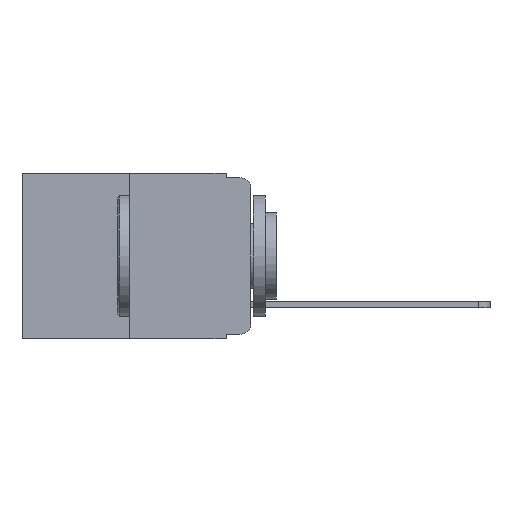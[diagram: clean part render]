
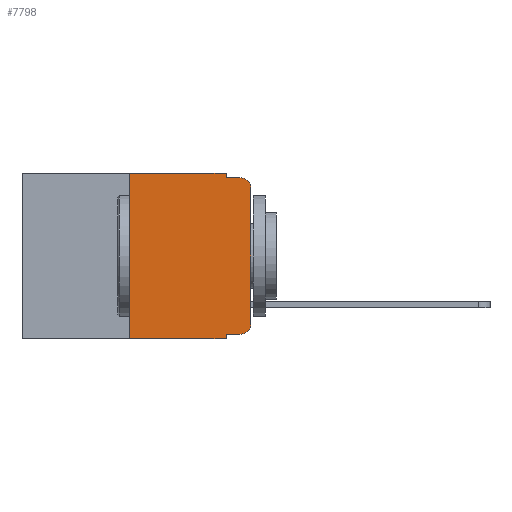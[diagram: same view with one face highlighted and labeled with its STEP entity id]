
A CAD part, left-side view. The second image highlights one B-rep face of the part: STEP entity #7798.
In plain terms, the highlighted planar face has unit normal (-1, 0, 0).
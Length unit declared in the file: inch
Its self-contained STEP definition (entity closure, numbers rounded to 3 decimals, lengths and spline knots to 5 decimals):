
#70 = DIRECTION ( 'NONE',  ( 0., 0., 1. ) ) ;
#279 = ORIENTED_EDGE ( 'NONE', *, *, #6738, .F. ) ;
#283 = CARTESIAN_POINT ( 'NONE',  ( 0., 0., 0. ) ) ;
#326 = EDGE_LOOP ( 'NONE', ( #13229, #1941, #5001, #279, #971, #1552, #1792, #2138, #4042, #7269 ) ) ;
#345 = VERTEX_POINT ( 'NONE', #1131 ) ;
#574 = CARTESIAN_POINT ( 'NONE',  ( 0., 0.051, -0.333 ) ) ;
#971 = ORIENTED_EDGE ( 'NONE', *, *, #5576, .F. ) ;
#1126 = EDGE_CURVE ( 'NONE', #345, #3323, #8335, .T. ) ;
#1131 = CARTESIAN_POINT ( 'NONE',  ( 0., 0.25, -0.343 ) ) ;
#1309 = VERTEX_POINT ( 'NONE', #3996 ) ;
#1339 = VERTEX_POINT ( 'NONE', #2635 ) ;
#1436 = CIRCLE ( 'NONE', #5843, 0.02 ) ;
#1552 = ORIENTED_EDGE ( 'NONE', *, *, #6776, .F. ) ;
#1668 = CIRCLE ( 'NONE', #12823, 0.02 ) ;
#1792 = ORIENTED_EDGE ( 'NONE', *, *, #1126, .T. ) ;
#1941 = ORIENTED_EDGE ( 'NONE', *, *, #6698, .T. ) ;
#2138 = ORIENTED_EDGE ( 'NONE', *, *, #6799, .F. ) ;
#2353 = DIRECTION ( 'NONE',  ( 0., -1., 0. ) ) ;
#2395 = DIRECTION ( 'NONE',  ( 1., 0., 0. ) ) ;
#2454 = VERTEX_POINT ( 'NONE', #9579 ) ;
#2459 = VERTEX_POINT ( 'NONE', #8147 ) ;
#2635 = CARTESIAN_POINT ( 'NONE',  ( 0., 0., -0.313 ) ) ;
#2829 = VERTEX_POINT ( 'NONE', #9335 ) ;
#3003 = VECTOR ( 'NONE', #8127, 39.37008 ) ;
#3323 = VERTEX_POINT ( 'NONE', #3618 ) ;
#3515 = DIRECTION ( 'NONE',  ( 0., 0., -1. ) ) ;
#3618 = CARTESIAN_POINT ( 'NONE',  ( 0., 0.051, -0.343 ) ) ;
#3692 = LINE ( 'NONE', #9010, #3003 ) ;
#3721 = DIRECTION ( 'NONE',  ( 0., -1., 0. ) ) ;
#3739 = CARTESIAN_POINT ( 'NONE',  ( 0., 0.051, 0. ) ) ;
#3996 = CARTESIAN_POINT ( 'NONE',  ( 0., 0.051, 0. ) ) ;
#4042 = ORIENTED_EDGE ( 'NONE', *, *, #6817, .T. ) ;
#4272 = VERTEX_POINT ( 'NONE', #6217 ) ;
#4340 = VERTEX_POINT ( 'NONE', #9428 ) ;
#4472 = CARTESIAN_POINT ( 'NONE',  ( 0., 0.473, 0. ) ) ;
#4518 = DIRECTION ( 'NONE',  ( 0., -1., 0. ) ) ;
#5001 = ORIENTED_EDGE ( 'NONE', *, *, #6722, .F. ) ;
#5290 = LINE ( 'NONE', #574, #12561 ) ;
#5558 = VECTOR ( 'NONE', #3721, 39.37008 ) ;
#5576 = EDGE_CURVE ( 'NONE', #2459, #1309, #8812, .T. ) ;
#5843 = AXIS2_PLACEMENT_3D ( 'NONE', #11190, #11175, #11147 ) ;
#6100 = VECTOR ( 'NONE', #4518, 39.37008 ) ;
#6217 = CARTESIAN_POINT ( 'NONE',  ( 0., 0.02, -0.01 ) ) ;
#6686 = EDGE_CURVE ( 'NONE', #1339, #2829, #10124, .T. ) ;
#6698 = EDGE_CURVE ( 'NONE', #2829, #4272, #1668, .T. ) ;
#6722 = EDGE_CURVE ( 'NONE', #4340, #4272, #11621, .T. ) ;
#6738 = EDGE_CURVE ( 'NONE', #1309, #4340, #8966, .T. ) ;
#6765 = CARTESIAN_POINT ( 'NONE',  ( 0., 0.473, 0. ) ) ;
#6776 = EDGE_CURVE ( 'NONE', #345, #2459, #3692, .T. ) ;
#6799 = EDGE_CURVE ( 'NONE', #6889, #3323, #13074, .T. ) ;
#6817 = EDGE_CURVE ( 'NONE', #6889, #2454, #5290, .T. ) ;
#6876 = EDGE_CURVE ( 'NONE', #2454, #1339, #1436, .T. ) ;
#6889 = VERTEX_POINT ( 'NONE', #11275 ) ;
#7269 = ORIENTED_EDGE ( 'NONE', *, *, #6876, .T. ) ;
#7657 = AXIS2_PLACEMENT_3D ( 'NONE', #6765, #2395, #9766 ) ;
#7798 = ADVANCED_FACE ( 'NONE', ( #8355 ), #8806, .F. ) ;
#8127 = DIRECTION ( 'NONE',  ( 0., 0., 1. ) ) ;
#8147 = CARTESIAN_POINT ( 'NONE',  ( 0., 0.25, 0. ) ) ;
#8335 = LINE ( 'NONE', #10536, #5558 ) ;
#8355 = FACE_OUTER_BOUND ( 'NONE', #326, .T. ) ;
#8806 = PLANE ( 'NONE',  #7657 ) ;
#8812 = LINE ( 'NONE', #4472, #6100 ) ;
#8966 = LINE ( 'NONE', #9173, #11332 ) ;
#9010 = CARTESIAN_POINT ( 'NONE',  ( 0., 0.25, 0. ) ) ;
#9173 = CARTESIAN_POINT ( 'NONE',  ( 0., 0.051, 0. ) ) ;
#9335 = CARTESIAN_POINT ( 'NONE',  ( 0., 0., -0.03 ) ) ;
#9377 = DIRECTION ( 'NONE',  ( 0., 0., -1. ) ) ;
#9428 = CARTESIAN_POINT ( 'NONE',  ( 0., 0.051, -0.01 ) ) ;
#9575 = VECTOR ( 'NONE', #10414, 39.37008 ) ;
#9579 = CARTESIAN_POINT ( 'NONE',  ( 0., 0.02, -0.333 ) ) ;
#9766 = DIRECTION ( 'NONE',  ( 0., 0., -1. ) ) ;
#10124 = LINE ( 'NONE', #283, #12144 ) ;
#10414 = DIRECTION ( 'NONE',  ( 0., -1., 0. ) ) ;
#10536 = CARTESIAN_POINT ( 'NONE',  ( 0., 0.473, -0.343 ) ) ;
#10559 = CARTESIAN_POINT ( 'NONE',  ( 0., 0.051, -0.01 ) ) ;
#10992 = DIRECTION ( 'NONE',  ( 0., 0., -1. ) ) ;
#11147 = DIRECTION ( 'NONE',  ( 0., 0., -1. ) ) ;
#11175 = DIRECTION ( 'NONE',  ( -1., 0., 0. ) ) ;
#11190 = CARTESIAN_POINT ( 'NONE',  ( 0., 0.02, -0.313 ) ) ;
#11211 = DIRECTION ( 'NONE',  ( -1., 0., 0. ) ) ;
#11275 = CARTESIAN_POINT ( 'NONE',  ( 0., 0.051, -0.333 ) ) ;
#11332 = VECTOR ( 'NONE', #9377, 39.37008 ) ;
#11621 = LINE ( 'NONE', #10559, #9575 ) ;
#12080 = CARTESIAN_POINT ( 'NONE',  ( 0., 0.02, -0.03 ) ) ;
#12144 = VECTOR ( 'NONE', #70, 39.37008 ) ;
#12561 = VECTOR ( 'NONE', #2353, 39.37008 ) ;
#12817 = VECTOR ( 'NONE', #3515, 39.37008 ) ;
#12823 = AXIS2_PLACEMENT_3D ( 'NONE', #12080, #11211, #10992 ) ;
#13074 = LINE ( 'NONE', #3739, #12817 ) ;
#13229 = ORIENTED_EDGE ( 'NONE', *, *, #6686, .T. ) ;
